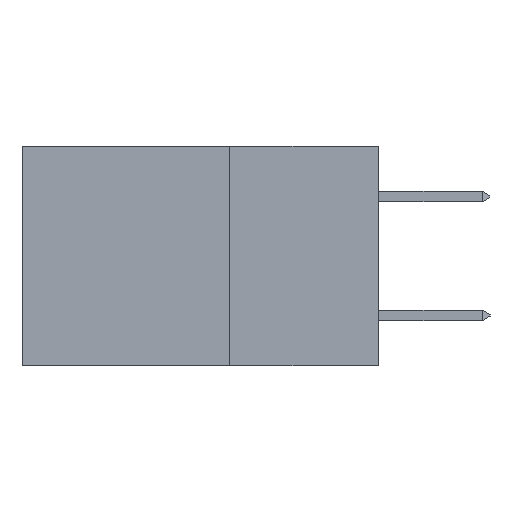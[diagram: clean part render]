
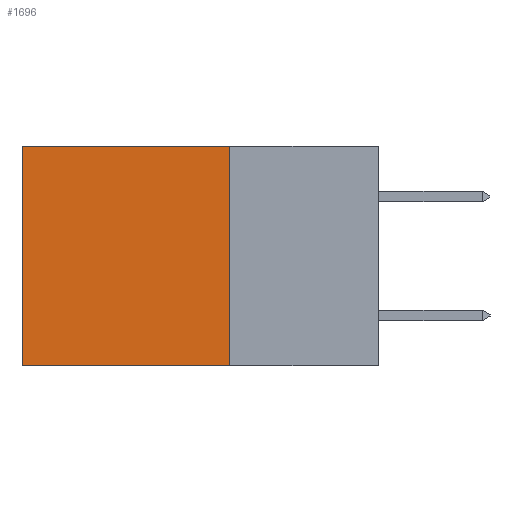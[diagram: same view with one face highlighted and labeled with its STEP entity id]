
A CAD part, left-side view. The second image highlights one B-rep face of the part: STEP entity #1696.
In plain terms, the highlighted planar face has unit normal (-1, 0, 0).
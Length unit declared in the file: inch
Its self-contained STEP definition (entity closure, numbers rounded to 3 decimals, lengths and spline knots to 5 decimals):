
#559 = EDGE_CURVE ( 'NONE', #694, #2170, #7980, .T. ) ;
#687 = DIRECTION ( 'NONE',  ( 0., 1., 0. ) ) ;
#694 = VERTEX_POINT ( 'NONE', #3636 ) ;
#1117 = EDGE_CURVE ( 'NONE', #8574, #3235, #5821, .T. ) ;
#1150 = LINE ( 'NONE', #5119, #4826 ) ;
#1326 = PLANE ( 'NONE',  #5361 ) ;
#1504 = FACE_OUTER_BOUND ( 'NONE', #3392, .T. ) ;
#1696 = ADVANCED_FACE ( 'NONE', ( #1504 ), #1326, .F. ) ;
#2170 = VERTEX_POINT ( 'NONE', #7214 ) ;
#2206 = VECTOR ( 'NONE', #5145, 39.37008 ) ;
#2245 = VECTOR ( 'NONE', #6933, 39.37008 ) ;
#2254 = CARTESIAN_POINT ( 'NONE',  ( 0.2615, 0.25, -0.37 ) ) ;
#2478 = CARTESIAN_POINT ( 'NONE',  ( 0.2615, 0.25, -0.37 ) ) ;
#3059 = DIRECTION ( 'NONE',  ( 1., 0., 0. ) ) ;
#3235 = VERTEX_POINT ( 'NONE', #8274 ) ;
#3392 = EDGE_LOOP ( 'NONE', ( #4008, #9025, #7259, #5372 ) ) ;
#3636 = CARTESIAN_POINT ( 'NONE',  ( 0.2615, 0.25, 0. ) ) ;
#4008 = ORIENTED_EDGE ( 'NONE', *, *, #1117, .T. ) ;
#4826 = VECTOR ( 'NONE', #687, 39.37008 ) ;
#5019 = EDGE_CURVE ( 'NONE', #2170, #3235, #8620, .T. ) ;
#5119 = CARTESIAN_POINT ( 'NONE',  ( 0.2615, 0.25, 0. ) ) ;
#5145 = DIRECTION ( 'NONE',  ( 0., 0., -1. ) ) ;
#5155 = CARTESIAN_POINT ( 'NONE',  ( 0.2615, 0.6, -0.37 ) ) ;
#5361 = AXIS2_PLACEMENT_3D ( 'NONE', #2254, #3059, #7550 ) ;
#5372 = ORIENTED_EDGE ( 'NONE', *, *, #8551, .T. ) ;
#5821 = LINE ( 'NONE', #5155, #2206 ) ;
#6680 = VECTOR ( 'NONE', #8417, 39.37008 ) ;
#6933 = DIRECTION ( 'NONE',  ( 0., 0., -1. ) ) ;
#7214 = CARTESIAN_POINT ( 'NONE',  ( 0.2615, 0.25, -0.37 ) ) ;
#7259 = ORIENTED_EDGE ( 'NONE', *, *, #559, .F. ) ;
#7379 = CARTESIAN_POINT ( 'NONE',  ( 0.2615, 0.25, -0.37 ) ) ;
#7550 = DIRECTION ( 'NONE',  ( 0., 0., -1. ) ) ;
#7724 = CARTESIAN_POINT ( 'NONE',  ( 0.2615, 0.6, 0. ) ) ;
#7980 = LINE ( 'NONE', #7379, #2245 ) ;
#8274 = CARTESIAN_POINT ( 'NONE',  ( 0.2615, 0.6, -0.37 ) ) ;
#8417 = DIRECTION ( 'NONE',  ( 0., 1., 0. ) ) ;
#8551 = EDGE_CURVE ( 'NONE', #694, #8574, #1150, .T. ) ;
#8574 = VERTEX_POINT ( 'NONE', #7724 ) ;
#8620 = LINE ( 'NONE', #2478, #6680 ) ;
#9025 = ORIENTED_EDGE ( 'NONE', *, *, #5019, .F. ) ;
